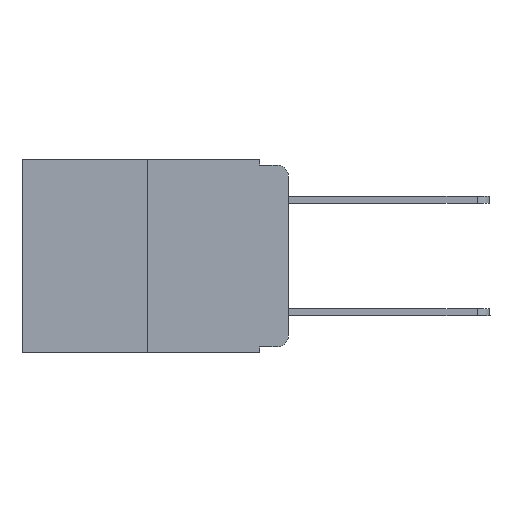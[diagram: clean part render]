
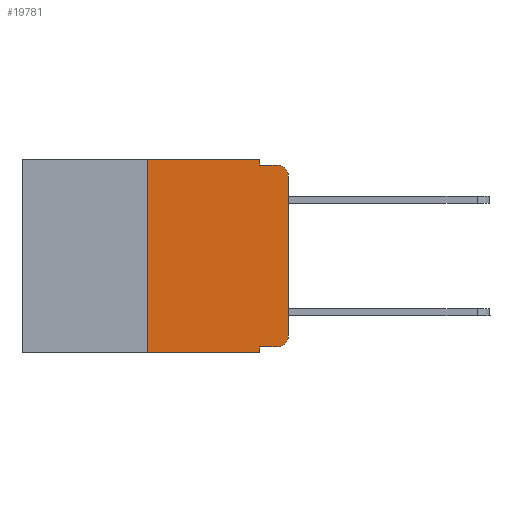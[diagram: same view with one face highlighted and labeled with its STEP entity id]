
A CAD part, left-side view. The second image highlights one B-rep face of the part: STEP entity #19781.
In plain terms, the highlighted planar face has unit normal (-1, 0, 0).
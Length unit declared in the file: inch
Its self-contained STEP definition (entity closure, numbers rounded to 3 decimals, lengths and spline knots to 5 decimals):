
#106 = VERTEX_POINT ( 'NONE', #13454 ) ;
#325 = DIRECTION ( 'NONE',  ( 0., -1., 0. ) ) ;
#976 = CIRCLE ( 'NONE', #2187, 0.02 ) ;
#1676 = FACE_OUTER_BOUND ( 'NONE', #23656, .T. ) ;
#2020 = ORIENTED_EDGE ( 'NONE', *, *, #19325, .F. ) ;
#2187 = AXIS2_PLACEMENT_3D ( 'NONE', #22758, #16472, #14802 ) ;
#3054 = VECTOR ( 'NONE', #6197, 39.37008 ) ;
#3055 = ORIENTED_EDGE ( 'NONE', *, *, #4508, .F. ) ;
#3461 = VECTOR ( 'NONE', #14177, 39.37008 ) ;
#3673 = DIRECTION ( 'NONE',  ( 0., -1., 0. ) ) ;
#4508 = EDGE_CURVE ( 'NONE', #22579, #11615, #14008, .T. ) ;
#4902 = CIRCLE ( 'NONE', #20125, 0.02 ) ;
#5120 = EDGE_CURVE ( 'NONE', #20639, #22579, #19223, .T. ) ;
#5173 = LINE ( 'NONE', #24668, #5973 ) ;
#5346 = CARTESIAN_POINT ( 'NONE',  ( 0., 0.02, -0.313 ) ) ;
#5973 = VECTOR ( 'NONE', #7230, 39.37008 ) ;
#6197 = DIRECTION ( 'NONE',  ( 0., -1., 0. ) ) ;
#7073 = VERTEX_POINT ( 'NONE', #18655 ) ;
#7230 = DIRECTION ( 'NONE',  ( 0., -1., 0. ) ) ;
#7361 = DIRECTION ( 'NONE',  ( 0., 0., -1. ) ) ;
#7617 = CARTESIAN_POINT ( 'NONE',  ( 0., 0.051, 0. ) ) ;
#7645 = VECTOR ( 'NONE', #7361, 39.37008 ) ;
#8130 = VECTOR ( 'NONE', #15130, 39.37008 ) ;
#9569 = ORIENTED_EDGE ( 'NONE', *, *, #20758, .F. ) ;
#9954 = ORIENTED_EDGE ( 'NONE', *, *, #15595, .T. ) ;
#10140 = VERTEX_POINT ( 'NONE', #11569 ) ;
#10146 = ORIENTED_EDGE ( 'NONE', *, *, #21787, .T. ) ;
#10571 = EDGE_CURVE ( 'NONE', #23156, #13789, #4902, .T. ) ;
#10750 = VERTEX_POINT ( 'NONE', #17979 ) ;
#10787 = LINE ( 'NONE', #20996, #18273 ) ;
#11322 = ORIENTED_EDGE ( 'NONE', *, *, #23005, .T. ) ;
#11494 = CARTESIAN_POINT ( 'NONE',  ( 0., 0.02, -0.333 ) ) ;
#11569 = CARTESIAN_POINT ( 'NONE',  ( 0., 0.051, -0.01 ) ) ;
#11615 = VERTEX_POINT ( 'NONE', #14039 ) ;
#12341 = LINE ( 'NONE', #18043, #24440 ) ;
#12750 = LINE ( 'NONE', #14449, #3461 ) ;
#13454 = CARTESIAN_POINT ( 'NONE',  ( 0., 0.051, -0.333 ) ) ;
#13506 = DIRECTION ( 'NONE',  ( -1., 0., 0. ) ) ;
#13753 = CARTESIAN_POINT ( 'NONE',  ( 0., 0.473, 0. ) ) ;
#13789 = VERTEX_POINT ( 'NONE', #24714 ) ;
#14008 = LINE ( 'NONE', #13753, #25340 ) ;
#14039 = CARTESIAN_POINT ( 'NONE',  ( 0., 0.051, 0. ) ) ;
#14177 = DIRECTION ( 'NONE',  ( 0., 0., 1. ) ) ;
#14445 = CARTESIAN_POINT ( 'NONE',  ( 0., 0.25, -0.343 ) ) ;
#14449 = CARTESIAN_POINT ( 'NONE',  ( 0., 0., 0. ) ) ;
#14802 = DIRECTION ( 'NONE',  ( 0., 0., -1. ) ) ;
#15130 = DIRECTION ( 'NONE',  ( 0., 0., 1. ) ) ;
#15333 = DIRECTION ( 'NONE',  ( 0., 0., -1. ) ) ;
#15595 = EDGE_CURVE ( 'NONE', #7073, #22623, #976, .T. ) ;
#15668 = LINE ( 'NONE', #7617, #7645 ) ;
#16472 = DIRECTION ( 'NONE',  ( -1., 0., 0. ) ) ;
#16626 = AXIS2_PLACEMENT_3D ( 'NONE', #21536, #21157, #17431 ) ;
#17156 = ORIENTED_EDGE ( 'NONE', *, *, #17764, .T. ) ;
#17431 = DIRECTION ( 'NONE',  ( 0., 0., -1. ) ) ;
#17764 = EDGE_CURVE ( 'NONE', #20639, #10750, #20285, .T. ) ;
#17979 = CARTESIAN_POINT ( 'NONE',  ( 0., 0.051, -0.343 ) ) ;
#17989 = CARTESIAN_POINT ( 'NONE',  ( 0., 0.473, -0.343 ) ) ;
#18043 = CARTESIAN_POINT ( 'NONE',  ( 0., 0.051, -0.01 ) ) ;
#18273 = VECTOR ( 'NONE', #20870, 39.37008 ) ;
#18655 = CARTESIAN_POINT ( 'NONE',  ( 0., 0., -0.03 ) ) ;
#18657 = CARTESIAN_POINT ( 'NONE',  ( 0., 0.25, 0. ) ) ;
#18811 = ORIENTED_EDGE ( 'NONE', *, *, #5120, .F. ) ;
#19105 = PLANE ( 'NONE',  #16626 ) ;
#19223 = LINE ( 'NONE', #20902, #8130 ) ;
#19325 = EDGE_CURVE ( 'NONE', #106, #10750, #15668, .T. ) ;
#19538 = CARTESIAN_POINT ( 'NONE',  ( 0., 0.02, -0.01 ) ) ;
#19781 = ADVANCED_FACE ( 'NONE', ( #1676 ), #19105, .F. ) ;
#20125 = AXIS2_PLACEMENT_3D ( 'NONE', #5346, #13506, #15333 ) ;
#20285 = LINE ( 'NONE', #17989, #3054 ) ;
#20552 = EDGE_CURVE ( 'NONE', #10140, #22623, #12341, .T. ) ;
#20639 = VERTEX_POINT ( 'NONE', #14445 ) ;
#20758 = EDGE_CURVE ( 'NONE', #11615, #10140, #10787, .T. ) ;
#20870 = DIRECTION ( 'NONE',  ( 0., 0., -1. ) ) ;
#20902 = CARTESIAN_POINT ( 'NONE',  ( 0., 0.25, 0. ) ) ;
#20996 = CARTESIAN_POINT ( 'NONE',  ( 0., 0.051, 0. ) ) ;
#21157 = DIRECTION ( 'NONE',  ( 1., 0., 0. ) ) ;
#21536 = CARTESIAN_POINT ( 'NONE',  ( 0., 0.473, 0. ) ) ;
#21787 = EDGE_CURVE ( 'NONE', #13789, #7073, #12750, .T. ) ;
#22579 = VERTEX_POINT ( 'NONE', #18657 ) ;
#22623 = VERTEX_POINT ( 'NONE', #19538 ) ;
#22758 = CARTESIAN_POINT ( 'NONE',  ( 0., 0.02, -0.03 ) ) ;
#23005 = EDGE_CURVE ( 'NONE', #106, #23156, #5173, .T. ) ;
#23156 = VERTEX_POINT ( 'NONE', #11494 ) ;
#23656 = EDGE_LOOP ( 'NONE', ( #10146, #9954, #23725, #9569, #3055, #18811, #17156, #2020, #11322, #24133 ) ) ;
#23725 = ORIENTED_EDGE ( 'NONE', *, *, #20552, .F. ) ;
#24133 = ORIENTED_EDGE ( 'NONE', *, *, #10571, .T. ) ;
#24440 = VECTOR ( 'NONE', #325, 39.37008 ) ;
#24668 = CARTESIAN_POINT ( 'NONE',  ( 0., 0.051, -0.333 ) ) ;
#24714 = CARTESIAN_POINT ( 'NONE',  ( 0., 0., -0.313 ) ) ;
#25340 = VECTOR ( 'NONE', #3673, 39.37008 ) ;
